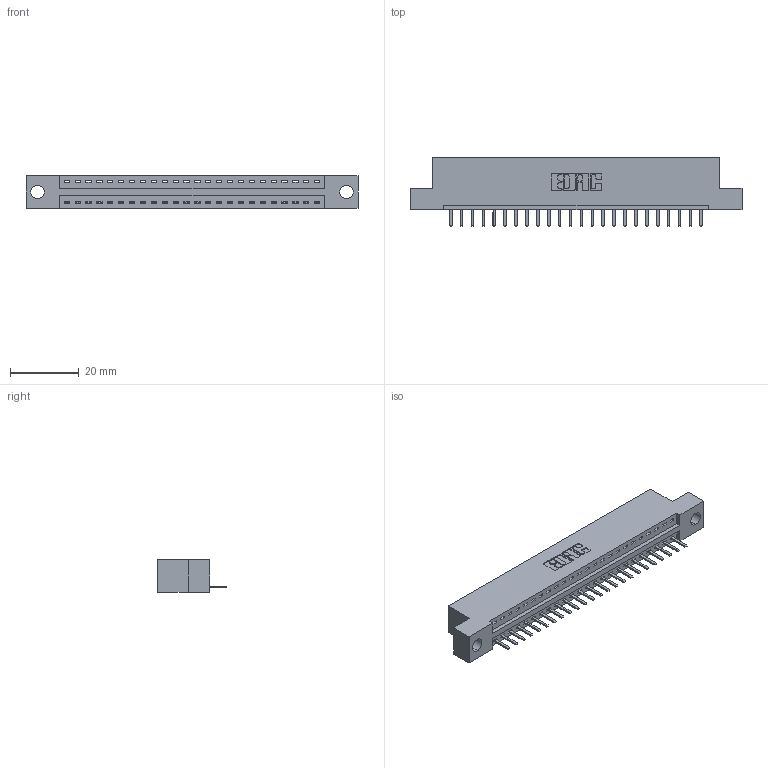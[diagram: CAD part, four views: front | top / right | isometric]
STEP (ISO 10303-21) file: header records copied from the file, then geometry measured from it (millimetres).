
FILE_DESCRIPTION (( 'STEP AP203' ), '1' );
FILE_NAME ('346-024-520-104.STEP', '2022-05-05T22:18:42', ( '' ), ( '' ), 'SwSTEP 2.0', 'SolidWorks 2020', '' );
FILE_SCHEMA (( 'CONFIG_CONTROL_DESIGN' ));
Length unit declared in the file: inch
Products named in the file (3): 346-024-520-104; 346 Part_Flush Mounting Lugs - 0.156 Dia-TH; 345-292-001_345-293-120
Assembly tree (25 placements, depth 2):
  346-024-520-104
    346 Part_Flush Mounting Lugs - 0.156 Dia-TH
    345-292-001_345-293-120  x24
Bounding box: 96.77 x 20.02 x 9.4 mm (x, y, z)
Volume: 8964.4 mm3; surface area: 10616.9 mm2
Topology: 25 solids, 25 shells, 1624 faces, 4781 edges, 3122 vertices
Faces by surface type: plane 1098, cylinder 526
Entity records: 17851 total; most frequent: CARTESIAN_POINT 3086, ORIENTED_EDGE 3030, DIRECTION 2731, EDGE_CURVE 1515, LINE 1283, VECTOR 1283, VERTEX_POINT 1006, AXIS2_PLACEMENT_3D 724
